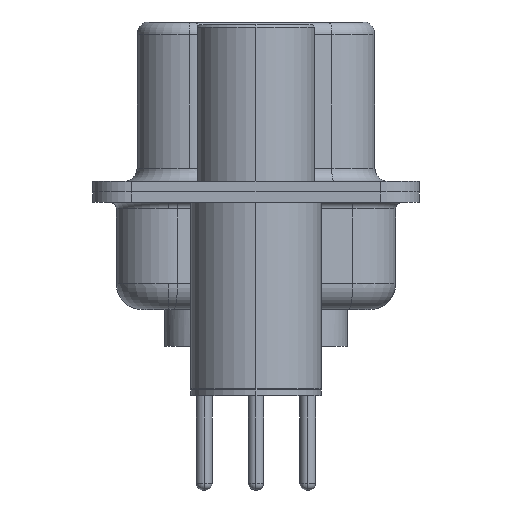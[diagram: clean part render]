
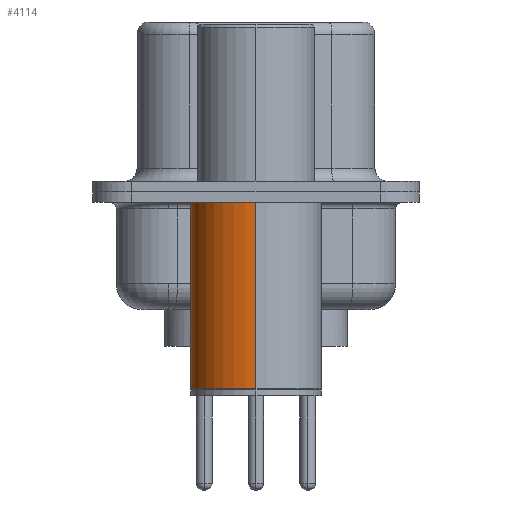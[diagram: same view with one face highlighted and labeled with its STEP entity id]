
A CAD part, left-side view. The second image highlights one B-rep face of the part: STEP entity #4114.
In plain terms, the highlighted cylindrical face has radius 2.5 mm (diameter 5 mm), a partial arc.
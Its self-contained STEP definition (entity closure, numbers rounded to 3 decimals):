
#1232 = EDGE_CURVE ( 'NONE', #2972, #1765, #5039, .T. ) ;
#1765 = VERTEX_POINT ( 'NONE', #17273 ) ;
#2848 = ORIENTED_EDGE ( 'NONE', *, *, #1232, .T. ) ;
#2972 = VERTEX_POINT ( 'NONE', #14763 ) ;
#3399 = CARTESIAN_POINT ( 'NONE',  ( -2.5, 0., 0.581 ) ) ;
#4114 = ADVANCED_FACE ( 'NONE', ( #17555 ), #28370, .T. ) ;
#4846 = CARTESIAN_POINT ( 'NONE',  ( 0., 0., -0.4 ) ) ;
#5039 = CIRCLE ( 'NONE', #5735, 2.5 ) ;
#5324 = AXIS2_PLACEMENT_3D ( 'NONE', #4846, #20141, #7118 ) ;
#5735 = AXIS2_PLACEMENT_3D ( 'NONE', #24824, #16424, #19633 ) ;
#5814 = EDGE_CURVE ( 'NONE', #1765, #24884, #18139, .T. ) ;
#6642 = EDGE_LOOP ( 'NONE', ( #2848, #25611, #10057, #15321 ) ) ;
#6941 = CIRCLE ( 'NONE', #5324, 2.5 ) ;
#7118 = DIRECTION ( 'NONE',  ( 1., 0., 0. ) ) ;
#7300 = DIRECTION ( 'NONE',  ( 0., 0., 1. ) ) ;
#7455 = CARTESIAN_POINT ( 'NONE',  ( 0., 0., 0.581 ) ) ;
#10057 = ORIENTED_EDGE ( 'NONE', *, *, #19914, .F. ) ;
#10482 = CARTESIAN_POINT ( 'NONE',  ( 2.5, 0., 0.581 ) ) ;
#11618 = AXIS2_PLACEMENT_3D ( 'NONE', #7455, #7300, #14998 ) ;
#13103 = VECTOR ( 'NONE', #25161, 1000. ) ;
#14596 = LINE ( 'NONE', #10482, #20977 ) ;
#14691 = EDGE_CURVE ( 'NONE', #2972, #16477, #14596, .T. ) ;
#14763 = CARTESIAN_POINT ( 'NONE',  ( 2.5, 0., -7.525 ) ) ;
#14998 = DIRECTION ( 'NONE',  ( 1., 0., 0. ) ) ;
#15321 = ORIENTED_EDGE ( 'NONE', *, *, #14691, .F. ) ;
#15506 = CARTESIAN_POINT ( 'NONE',  ( 2.5, 0., -0.4 ) ) ;
#16424 = DIRECTION ( 'NONE',  ( 0., 0., 1. ) ) ;
#16477 = VERTEX_POINT ( 'NONE', #15506 ) ;
#16525 = CARTESIAN_POINT ( 'NONE',  ( -2.5, 0., -0.4 ) ) ;
#17273 = CARTESIAN_POINT ( 'NONE',  ( -2.5, 0., -7.525 ) ) ;
#17555 = FACE_OUTER_BOUND ( 'NONE', #6642, .T. ) ;
#18139 = LINE ( 'NONE', #3399, #13103 ) ;
#19633 = DIRECTION ( 'NONE',  ( 1., 0., 0. ) ) ;
#19914 = EDGE_CURVE ( 'NONE', #16477, #24884, #6941, .T. ) ;
#20141 = DIRECTION ( 'NONE',  ( 0., 0., 1. ) ) ;
#20977 = VECTOR ( 'NONE', #23363, 1000. ) ;
#23363 = DIRECTION ( 'NONE',  ( 0., 0., 1. ) ) ;
#24824 = CARTESIAN_POINT ( 'NONE',  ( 0., 0., -7.525 ) ) ;
#24884 = VERTEX_POINT ( 'NONE', #16525 ) ;
#25161 = DIRECTION ( 'NONE',  ( 0., 0., 1. ) ) ;
#25611 = ORIENTED_EDGE ( 'NONE', *, *, #5814, .T. ) ;
#28370 = CYLINDRICAL_SURFACE ( 'NONE', #11618, 2.5 ) ;
